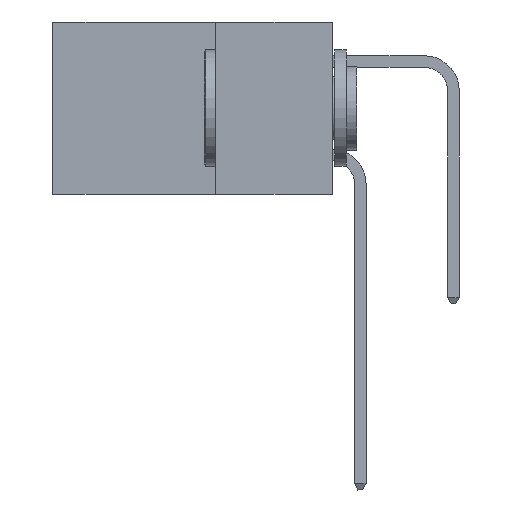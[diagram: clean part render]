
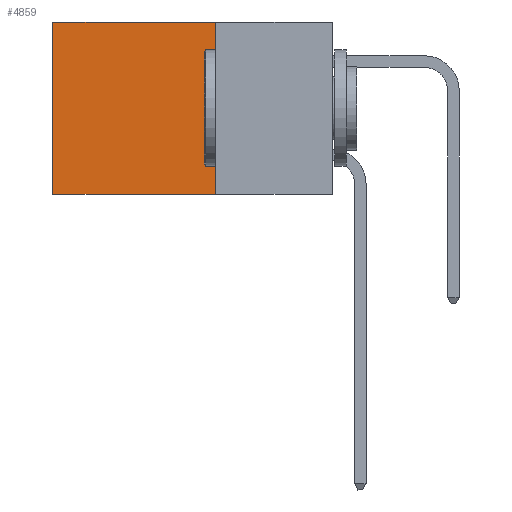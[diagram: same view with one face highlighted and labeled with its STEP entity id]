
A CAD part, left-side view. The second image highlights one B-rep face of the part: STEP entity #4859.
In plain terms, the highlighted planar face has unit normal (-1, 0, 0).
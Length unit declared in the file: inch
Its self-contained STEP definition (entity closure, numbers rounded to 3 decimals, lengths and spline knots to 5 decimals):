
#305 = LINE ( 'NONE', #25248, #20562 ) ;
#437 = LINE ( 'NONE', #4420, #25268 ) ;
#1484 = AXIS2_PLACEMENT_3D ( 'NONE', #4868, #4782, #4778 ) ;
#1578 = LINE ( 'NONE', #21860, #11430 ) ;
#3786 = EDGE_CURVE ( 'NONE', #20666, #24274, #5499, .T. ) ;
#4420 = CARTESIAN_POINT ( 'NONE',  ( 0.2615, 0.25, -0.37 ) ) ;
#4778 = DIRECTION ( 'NONE',  ( 0., 0., -1. ) ) ;
#4782 = DIRECTION ( 'NONE',  ( 1., 0., 0. ) ) ;
#4859 = ADVANCED_FACE ( 'NONE', ( #23803 ), #4897, .F. ) ;
#4868 = CARTESIAN_POINT ( 'NONE',  ( 0.2615, 0.25, -0.37 ) ) ;
#4892 = VECTOR ( 'NONE', #6199, 39.37008 ) ;
#4897 = PLANE ( 'NONE',  #1484 ) ;
#5499 = LINE ( 'NONE', #6632, #4892 ) ;
#6134 = CARTESIAN_POINT ( 'NONE',  ( 0.2615, 0.25, -0.37 ) ) ;
#6199 = DIRECTION ( 'NONE',  ( 0., 0., -1. ) ) ;
#6632 = CARTESIAN_POINT ( 'NONE',  ( 0.2615, 0.6, -0.37 ) ) ;
#8361 = ORIENTED_EDGE ( 'NONE', *, *, #3786, .T. ) ;
#8375 = DIRECTION ( 'NONE',  ( 0., 0., -1. ) ) ;
#9628 = DIRECTION ( 'NONE',  ( 0., 1., 0. ) ) ;
#11430 = VECTOR ( 'NONE', #19904, 39.37008 ) ;
#11968 = VERTEX_POINT ( 'NONE', #6134 ) ;
#12359 = CARTESIAN_POINT ( 'NONE',  ( 0.2615, 0.25, 0. ) ) ;
#14047 = EDGE_CURVE ( 'NONE', #11968, #24274, #1578, .T. ) ;
#14551 = EDGE_CURVE ( 'NONE', #24417, #20666, #305, .T. ) ;
#15717 = ORIENTED_EDGE ( 'NONE', *, *, #17970, .F. ) ;
#15888 = CARTESIAN_POINT ( 'NONE',  ( 0.2615, 0.6, -0.37 ) ) ;
#17748 = CARTESIAN_POINT ( 'NONE',  ( 0.2615, 0.6, 0. ) ) ;
#17970 = EDGE_CURVE ( 'NONE', #24417, #11968, #437, .T. ) ;
#18788 = EDGE_LOOP ( 'NONE', ( #8361, #20838, #15717, #21345 ) ) ;
#19904 = DIRECTION ( 'NONE',  ( 0., 1., 0. ) ) ;
#20562 = VECTOR ( 'NONE', #9628, 39.37008 ) ;
#20666 = VERTEX_POINT ( 'NONE', #17748 ) ;
#20838 = ORIENTED_EDGE ( 'NONE', *, *, #14047, .F. ) ;
#21345 = ORIENTED_EDGE ( 'NONE', *, *, #14551, .T. ) ;
#21860 = CARTESIAN_POINT ( 'NONE',  ( 0.2615, 0.25, -0.37 ) ) ;
#23803 = FACE_OUTER_BOUND ( 'NONE', #18788, .T. ) ;
#24274 = VERTEX_POINT ( 'NONE', #15888 ) ;
#24417 = VERTEX_POINT ( 'NONE', #12359 ) ;
#25248 = CARTESIAN_POINT ( 'NONE',  ( 0.2615, 0.25, 0. ) ) ;
#25268 = VECTOR ( 'NONE', #8375, 39.37008 ) ;
